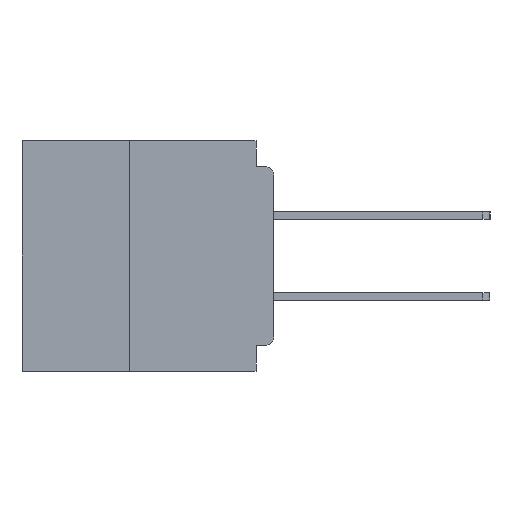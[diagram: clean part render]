
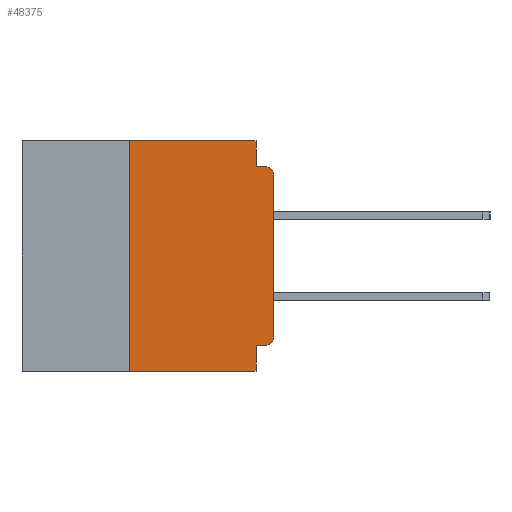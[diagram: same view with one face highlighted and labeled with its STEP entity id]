
A CAD part, left-side view. The second image highlights one B-rep face of the part: STEP entity #48375.
In plain terms, the highlighted planar face has unit normal (-1, 0, 0).
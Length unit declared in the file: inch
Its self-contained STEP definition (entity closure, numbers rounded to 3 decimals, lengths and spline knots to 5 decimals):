
#55 = ORIENTED_EDGE ( 'NONE', *, *, #1128, .F. ) ;
#199 = AXIS2_PLACEMENT_3D ( 'NONE', #26948, #836, #31316 ) ;
#590 = ORIENTED_EDGE ( 'NONE', *, *, #34317, .T. ) ;
#836 = DIRECTION ( 'NONE',  ( 1., 0., 0. ) ) ;
#1128 = EDGE_CURVE ( 'NONE', #4061, #55210, #4795, .T. ) ;
#1181 = VERTEX_POINT ( 'NONE', #43777 ) ;
#1296 = CARTESIAN_POINT ( 'NONE',  ( 0., 0.25, -0.4 ) ) ;
#1476 = EDGE_CURVE ( 'NONE', #39155, #48755, #31994, .T. ) ;
#1541 = EDGE_CURVE ( 'NONE', #53173, #39265, #50911, .T. ) ;
#2000 = VECTOR ( 'NONE', #23118, 39.37008 ) ;
#2135 = CIRCLE ( 'NONE', #36790, 0.015 ) ;
#4061 = VERTEX_POINT ( 'NONE', #20796 ) ;
#4328 = ORIENTED_EDGE ( 'NONE', *, *, #1476, .T. ) ;
#4795 = LINE ( 'NONE', #1296, #49601 ) ;
#5512 = CARTESIAN_POINT ( 'NONE',  ( 0., 0., -0.045 ) ) ;
#6332 = VERTEX_POINT ( 'NONE', #12731 ) ;
#6922 = CARTESIAN_POINT ( 'NONE',  ( 0., 0.437, -0.4 ) ) ;
#7463 = FACE_OUTER_BOUND ( 'NONE', #51635, .T. ) ;
#8007 = EDGE_CURVE ( 'NONE', #48755, #25916, #16136, .T. ) ;
#9298 = ORIENTED_EDGE ( 'NONE', *, *, #8007, .T. ) ;
#11101 = EDGE_CURVE ( 'NONE', #55210, #32825, #50375, .T. ) ;
#12731 = CARTESIAN_POINT ( 'NONE',  ( 0., 0.031, -0.4 ) ) ;
#12901 = CARTESIAN_POINT ( 'NONE',  ( 0., 0.031, -0.045 ) ) ;
#13141 = DIRECTION ( 'NONE',  ( 0., 0., -1. ) ) ;
#14939 = LINE ( 'NONE', #36068, #2000 ) ;
#15674 = CARTESIAN_POINT ( 'NONE',  ( 0., 0.015, -0.34 ) ) ;
#15747 = VECTOR ( 'NONE', #30898, 39.37008 ) ;
#16136 = LINE ( 'NONE', #27155, #37954 ) ;
#18167 = PLANE ( 'NONE',  #199 ) ;
#19135 = DIRECTION ( 'NONE',  ( -1., 0., 0. ) ) ;
#20447 = CARTESIAN_POINT ( 'NONE',  ( 0., 0., -0.06 ) ) ;
#20779 = DIRECTION ( 'NONE',  ( 0., -1., 0. ) ) ;
#20796 = CARTESIAN_POINT ( 'NONE',  ( 0., 0.25, -0.4 ) ) ;
#21487 = CARTESIAN_POINT ( 'NONE',  ( 0., 0.015, -0.355 ) ) ;
#21537 = ORIENTED_EDGE ( 'NONE', *, *, #1541, .F. ) ;
#22243 = CARTESIAN_POINT ( 'NONE',  ( 0., 0.015, -0.045 ) ) ;
#22315 = DIRECTION ( 'NONE',  ( 0., 0., -1. ) ) ;
#23118 = DIRECTION ( 'NONE',  ( 0., 1., 0. ) ) ;
#23794 = DIRECTION ( 'NONE',  ( 0., 0., 1. ) ) ;
#24467 = DIRECTION ( 'NONE',  ( 0., -1., 0. ) ) ;
#25720 = EDGE_CURVE ( 'NONE', #25916, #39265, #2135, .T. ) ;
#25916 = VERTEX_POINT ( 'NONE', #20447 ) ;
#25964 = CARTESIAN_POINT ( 'NONE',  ( 0., 0.031, 0. ) ) ;
#26948 = CARTESIAN_POINT ( 'NONE',  ( 0., 0.437, 0. ) ) ;
#27155 = CARTESIAN_POINT ( 'NONE',  ( 0., 0., 0. ) ) ;
#27825 = VECTOR ( 'NONE', #24467, 39.37008 ) ;
#28158 = VECTOR ( 'NONE', #22315, 39.37008 ) ;
#30898 = DIRECTION ( 'NONE',  ( 0., -1., 0. ) ) ;
#30945 = ORIENTED_EDGE ( 'NONE', *, *, #11101, .F. ) ;
#31064 = CARTESIAN_POINT ( 'NONE',  ( 0., 0.031, 0. ) ) ;
#31316 = DIRECTION ( 'NONE',  ( 0., 0., -1. ) ) ;
#31994 = CIRCLE ( 'NONE', #52592, 0.015 ) ;
#32825 = VERTEX_POINT ( 'NONE', #25964 ) ;
#33842 = LINE ( 'NONE', #42990, #45371 ) ;
#34317 = EDGE_CURVE ( 'NONE', #4061, #6332, #39403, .T. ) ;
#35284 = CARTESIAN_POINT ( 'NONE',  ( 0., 0.437, 0. ) ) ;
#36068 = CARTESIAN_POINT ( 'NONE',  ( 0., 0., -0.355 ) ) ;
#36312 = ORIENTED_EDGE ( 'NONE', *, *, #47485, .F. ) ;
#36790 = AXIS2_PLACEMENT_3D ( 'NONE', #45193, #19135, #49451 ) ;
#37954 = VECTOR ( 'NONE', #53053, 39.37008 ) ;
#38610 = EDGE_CURVE ( 'NONE', #32825, #53173, #41053, .T. ) ;
#39155 = VERTEX_POINT ( 'NONE', #21487 ) ;
#39265 = VERTEX_POINT ( 'NONE', #22243 ) ;
#39403 = LINE ( 'NONE', #6922, #27825 ) ;
#39475 = VECTOR ( 'NONE', #20779, 39.37008 ) ;
#41053 = LINE ( 'NONE', #31064, #28158 ) ;
#42473 = ORIENTED_EDGE ( 'NONE', *, *, #25720, .T. ) ;
#42990 = CARTESIAN_POINT ( 'NONE',  ( 0., 0.031, -0.4 ) ) ;
#43777 = CARTESIAN_POINT ( 'NONE',  ( 0., 0.031, -0.355 ) ) ;
#44526 = ORIENTED_EDGE ( 'NONE', *, *, #38610, .F. ) ;
#45038 = CARTESIAN_POINT ( 'NONE',  ( 0., 0.25, 0. ) ) ;
#45193 = CARTESIAN_POINT ( 'NONE',  ( 0., 0.015, -0.06 ) ) ;
#45371 = VECTOR ( 'NONE', #47339, 39.37008 ) ;
#45668 = ORIENTED_EDGE ( 'NONE', *, *, #48451, .F. ) ;
#46124 = DIRECTION ( 'NONE',  ( -1., 0., 0. ) ) ;
#47339 = DIRECTION ( 'NONE',  ( 0., 0., -1. ) ) ;
#47485 = EDGE_CURVE ( 'NONE', #1181, #6332, #33842, .T. ) ;
#48375 = ADVANCED_FACE ( 'NONE', ( #7463 ), #18167, .F. ) ;
#48451 = EDGE_CURVE ( 'NONE', #39155, #1181, #14939, .T. ) ;
#48755 = VERTEX_POINT ( 'NONE', #50939 ) ;
#49451 = DIRECTION ( 'NONE',  ( 0., 0., -1. ) ) ;
#49601 = VECTOR ( 'NONE', #23794, 39.37008 ) ;
#50375 = LINE ( 'NONE', #35284, #15747 ) ;
#50911 = LINE ( 'NONE', #5512, #39475 ) ;
#50939 = CARTESIAN_POINT ( 'NONE',  ( 0., 0., -0.34 ) ) ;
#51635 = EDGE_LOOP ( 'NONE', ( #9298, #42473, #21537, #44526, #30945, #55, #590, #36312, #45668, #4328 ) ) ;
#52592 = AXIS2_PLACEMENT_3D ( 'NONE', #15674, #46124, #13141 ) ;
#53053 = DIRECTION ( 'NONE',  ( 0., 0., 1. ) ) ;
#53173 = VERTEX_POINT ( 'NONE', #12901 ) ;
#55210 = VERTEX_POINT ( 'NONE', #45038 ) ;
